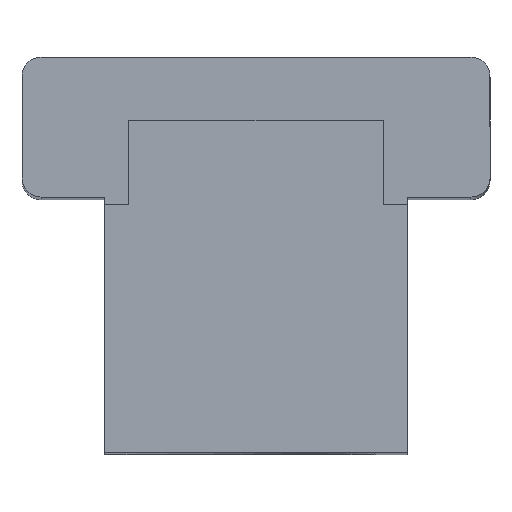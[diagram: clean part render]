
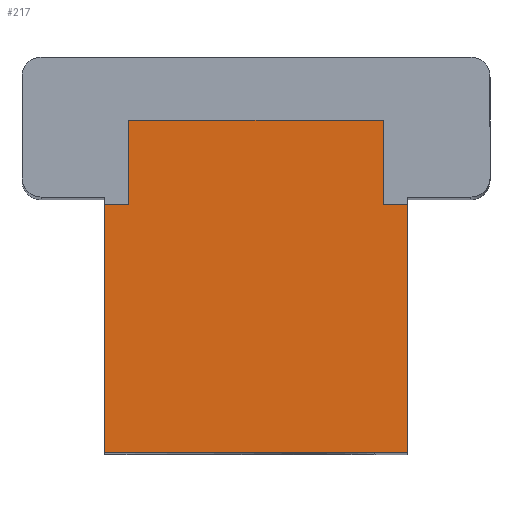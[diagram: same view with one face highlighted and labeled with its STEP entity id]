
A CAD part, top view. The second image highlights one B-rep face of the part: STEP entity #217.
In plain terms, the highlighted planar face has unit normal (0, 0, 1).
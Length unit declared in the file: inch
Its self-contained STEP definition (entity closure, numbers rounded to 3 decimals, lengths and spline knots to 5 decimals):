
#41 = CARTESIAN_POINT ( 'NONE',  ( 0.2, 1.182, 2.4 ) ) ;
#73 = CARTESIAN_POINT ( 'NONE',  ( 0.238, 0.66, 2.4 ) ) ;
#77 = ORIENTED_EDGE ( 'NONE', *, *, #1378, .T. ) ;
#116 = CARTESIAN_POINT ( 'NONE',  ( -0.238, 1.062, 2.4 ) ) ;
#117 = VERTEX_POINT ( 'NONE', #1133 ) ;
#217 = ADVANCED_FACE ( 'NONE', ( #1153 ), #2290, .T. ) ;
#225 = LINE ( 'NONE', #2096, #1933 ) ;
#275 = DIRECTION ( 'NONE',  ( 0., 1., 0. ) ) ;
#329 = EDGE_CURVE ( 'NONE', #913, #117, #1623, .T. ) ;
#355 = VERTEX_POINT ( 'NONE', #903 ) ;
#385 = ORIENTED_EDGE ( 'NONE', *, *, #1901, .T. ) ;
#393 = ORIENTED_EDGE ( 'NONE', *, *, #1100, .F. ) ;
#431 = ORIENTED_EDGE ( 'NONE', *, *, #2417, .F. ) ;
#470 = CARTESIAN_POINT ( 'NONE',  ( 0.238, 0.66, 2.4 ) ) ;
#484 = DIRECTION ( 'NONE',  ( 1., 0., 0. ) ) ;
#558 = CARTESIAN_POINT ( 'NONE',  ( 0.2, 1.05, 2.4 ) ) ;
#574 = DIRECTION ( 'NONE',  ( 0., 0., 1. ) ) ;
#668 = CARTESIAN_POINT ( 'NONE',  ( 0.238, 0.66, 2.4 ) ) ;
#812 = VERTEX_POINT ( 'NONE', #558 ) ;
#813 = DIRECTION ( 'NONE',  ( 1., 0., 0. ) ) ;
#823 = EDGE_LOOP ( 'NONE', ( #431, #393, #1173, #385, #1445, #2104, #2157, #77 ) ) ;
#859 = CARTESIAN_POINT ( 'NONE',  ( -0.2, 1.182, 2.4 ) ) ;
#903 = CARTESIAN_POINT ( 'NONE',  ( -0.238, 1.05, 2.4 ) ) ;
#913 = VERTEX_POINT ( 'NONE', #470 ) ;
#1009 = LINE ( 'NONE', #1997, #2334 ) ;
#1015 = CARTESIAN_POINT ( 'NONE',  ( -0.2, 1.05, 2.4 ) ) ;
#1078 = EDGE_CURVE ( 'NONE', #2405, #913, #1605, .T. ) ;
#1100 = EDGE_CURVE ( 'NONE', #1339, #1392, #2167, .T. ) ;
#1133 = CARTESIAN_POINT ( 'NONE',  ( 0.238, 1.05, 2.4 ) ) ;
#1153 = FACE_OUTER_BOUND ( 'NONE', #823, .T. ) ;
#1161 = LINE ( 'NONE', #1342, #1576 ) ;
#1173 = ORIENTED_EDGE ( 'NONE', *, *, #2283, .T. ) ;
#1174 = DIRECTION ( 'NONE',  ( -1., 0., 0. ) ) ;
#1183 = AXIS2_PLACEMENT_3D ( 'NONE', #1335, #574, #1912 ) ;
#1202 = CARTESIAN_POINT ( 'NONE',  ( -0.238, 0.66, 2.4 ) ) ;
#1219 = CARTESIAN_POINT ( 'NONE',  ( 0.2, 1.05, 2.4 ) ) ;
#1232 = DIRECTION ( 'NONE',  ( 0., 1., 0. ) ) ;
#1335 = CARTESIAN_POINT ( 'NONE',  ( -0.338, 1.092, 2.4 ) ) ;
#1339 = VERTEX_POINT ( 'NONE', #2449 ) ;
#1342 = CARTESIAN_POINT ( 'NONE',  ( -0.338, 1.05, 2.4 ) ) ;
#1378 = EDGE_CURVE ( 'NONE', #812, #1403, #1745, .T. ) ;
#1392 = VERTEX_POINT ( 'NONE', #859 ) ;
#1403 = VERTEX_POINT ( 'NONE', #41 ) ;
#1419 = VECTOR ( 'NONE', #275, 39.37008 ) ;
#1430 = LINE ( 'NONE', #116, #2133 ) ;
#1445 = ORIENTED_EDGE ( 'NONE', *, *, #1078, .T. ) ;
#1576 = VECTOR ( 'NONE', #2085, 39.37008 ) ;
#1605 = LINE ( 'NONE', #668, #1830 ) ;
#1623 = LINE ( 'NONE', #73, #1419 ) ;
#1701 = VECTOR ( 'NONE', #1232, 39.37008 ) ;
#1745 = LINE ( 'NONE', #1219, #2352 ) ;
#1807 = DIRECTION ( 'NONE',  ( 0., -1., 0. ) ) ;
#1830 = VECTOR ( 'NONE', #484, 39.37008 ) ;
#1901 = EDGE_CURVE ( 'NONE', #355, #2405, #1430, .T. ) ;
#1912 = DIRECTION ( 'NONE',  ( 1., 0., 0. ) ) ;
#1933 = VECTOR ( 'NONE', #1174, 39.37008 ) ;
#1962 = DIRECTION ( 'NONE',  ( 0., 1., 0. ) ) ;
#1997 = CARTESIAN_POINT ( 'NONE',  ( -0.2, 1.182, 2.4 ) ) ;
#2085 = DIRECTION ( 'NONE',  ( 1., 0., 0. ) ) ;
#2096 = CARTESIAN_POINT ( 'NONE',  ( -0.338, 1.05, 2.4 ) ) ;
#2104 = ORIENTED_EDGE ( 'NONE', *, *, #329, .T. ) ;
#2133 = VECTOR ( 'NONE', #1807, 39.37008 ) ;
#2157 = ORIENTED_EDGE ( 'NONE', *, *, #2321, .F. ) ;
#2167 = LINE ( 'NONE', #1015, #1701 ) ;
#2283 = EDGE_CURVE ( 'NONE', #1339, #355, #225, .T. ) ;
#2290 = PLANE ( 'NONE',  #1183 ) ;
#2321 = EDGE_CURVE ( 'NONE', #812, #117, #1161, .T. ) ;
#2334 = VECTOR ( 'NONE', #813, 39.37008 ) ;
#2352 = VECTOR ( 'NONE', #1962, 39.37008 ) ;
#2405 = VERTEX_POINT ( 'NONE', #1202 ) ;
#2417 = EDGE_CURVE ( 'NONE', #1392, #1403, #1009, .T. ) ;
#2449 = CARTESIAN_POINT ( 'NONE',  ( -0.2, 1.05, 2.4 ) ) ;
